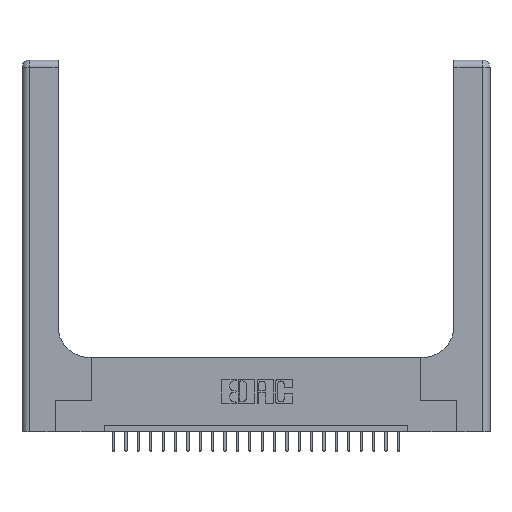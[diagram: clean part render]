
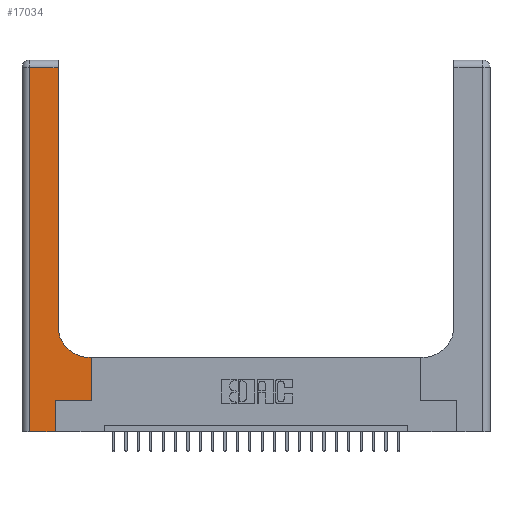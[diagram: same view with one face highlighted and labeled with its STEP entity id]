
A CAD part, top view. The second image highlights one B-rep face of the part: STEP entity #17034.
In plain terms, the highlighted planar face has unit normal (0, 0, 1).
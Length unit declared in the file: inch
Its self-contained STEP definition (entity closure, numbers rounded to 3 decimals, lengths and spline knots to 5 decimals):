
#366 = LINE ( 'NONE', #868, #18092 ) ;
#513 = DIRECTION ( 'NONE',  ( 0., 1., 0. ) ) ;
#868 = CARTESIAN_POINT ( 'NONE',  ( 0., 2.94, 0.37 ) ) ;
#1115 = EDGE_CURVE ( 'NONE', #24318, #11348, #1898, .T. ) ;
#1145 = VERTEX_POINT ( 'NONE', #16154 ) ;
#1175 = PLANE ( 'NONE',  #11330 ) ;
#1395 = LINE ( 'NONE', #10320, #18798 ) ;
#1799 = VECTOR ( 'NONE', #15553, 39.37008 ) ;
#1898 = LINE ( 'NONE', #23391, #19881 ) ;
#1941 = VERTEX_POINT ( 'NONE', #11925 ) ;
#1975 = CARTESIAN_POINT ( 'NONE',  ( 0.06, 2.94, 0.37 ) ) ;
#2392 = VERTEX_POINT ( 'NONE', #14269 ) ;
#2395 = CARTESIAN_POINT ( 'NONE',  ( 0.5415, 0.6, 0.37 ) ) ;
#2659 = ORIENTED_EDGE ( 'NONE', *, *, #9084, .T. ) ;
#3043 = LINE ( 'NONE', #3652, #1799 ) ;
#3112 = ORIENTED_EDGE ( 'NONE', *, *, #6269, .T. ) ;
#3192 = CIRCLE ( 'NONE', #4541, 0.25 ) ;
#3473 = CARTESIAN_POINT ( 'NONE',  ( 0.269, 0.25, 0.37 ) ) ;
#3652 = CARTESIAN_POINT ( 'NONE',  ( 0.269, 0., 0.37 ) ) ;
#3776 = CARTESIAN_POINT ( 'NONE',  ( 0., 0., 0.37 ) ) ;
#4541 = AXIS2_PLACEMENT_3D ( 'NONE', #4554, #4646, #24519 ) ;
#4554 = CARTESIAN_POINT ( 'NONE',  ( 0.5415, 0.85, 0.37 ) ) ;
#4646 = DIRECTION ( 'NONE',  ( 0., 0., -1. ) ) ;
#4656 = ORIENTED_EDGE ( 'NONE', *, *, #1115, .T. ) ;
#5055 = CARTESIAN_POINT ( 'NONE',  ( 0.5585, 0.25, 0.37 ) ) ;
#5147 = CARTESIAN_POINT ( 'NONE',  ( 0.2915, 0.6, 0.37 ) ) ;
#5500 = ORIENTED_EDGE ( 'NONE', *, *, #11377, .T. ) ;
#6269 = EDGE_CURVE ( 'NONE', #19962, #1941, #1395, .T. ) ;
#7213 = DIRECTION ( 'NONE',  ( 0., 1., 0. ) ) ;
#7850 = LINE ( 'NONE', #3776, #21528 ) ;
#7855 = VECTOR ( 'NONE', #7213, 39.37008 ) ;
#8507 = ORIENTED_EDGE ( 'NONE', *, *, #16821, .T. ) ;
#9084 = EDGE_CURVE ( 'NONE', #22140, #24662, #3192, .T. ) ;
#9133 = DIRECTION ( 'NONE',  ( 1., 0., 0. ) ) ;
#10320 = CARTESIAN_POINT ( 'NONE',  ( 0.5585, 0.25, 0.37 ) ) ;
#11205 = EDGE_LOOP ( 'NONE', ( #14551, #14239, #4656, #8507, #25707, #5500, #3112, #23960, #2659 ) ) ;
#11330 = AXIS2_PLACEMENT_3D ( 'NONE', #13000, #16996, #24773 ) ;
#11348 = VERTEX_POINT ( 'NONE', #12780 ) ;
#11377 = EDGE_CURVE ( 'NONE', #2392, #19962, #21696, .T. ) ;
#11525 = DIRECTION ( 'NONE',  ( 1., 0., 0. ) ) ;
#11925 = CARTESIAN_POINT ( 'NONE',  ( 0.5585, 0.6, 0.37 ) ) ;
#12433 = EDGE_CURVE ( 'NONE', #1145, #2392, #3043, .T. ) ;
#12780 = CARTESIAN_POINT ( 'NONE',  ( 0.06, 0., 0.37 ) ) ;
#12856 = DIRECTION ( 'NONE',  ( -1., 0., 0. ) ) ;
#13000 = CARTESIAN_POINT ( 'NONE',  ( 0., 3., 0.37 ) ) ;
#13415 = CARTESIAN_POINT ( 'NONE',  ( 0.2915, 2.94, 0.37 ) ) ;
#13504 = FACE_OUTER_BOUND ( 'NONE', #11205, .T. ) ;
#14239 = ORIENTED_EDGE ( 'NONE', *, *, #17835, .T. ) ;
#14269 = CARTESIAN_POINT ( 'NONE',  ( 0.269, 0.25, 0.37 ) ) ;
#14551 = ORIENTED_EDGE ( 'NONE', *, *, #22501, .T. ) ;
#14830 = DIRECTION ( 'NONE',  ( -1., 0., 0. ) ) ;
#15553 = DIRECTION ( 'NONE',  ( 0., 1., 0. ) ) ;
#16154 = CARTESIAN_POINT ( 'NONE',  ( 0.269, 0., 0.37 ) ) ;
#16480 = VECTOR ( 'NONE', #9133, 39.37008 ) ;
#16821 = EDGE_CURVE ( 'NONE', #11348, #1145, #7850, .T. ) ;
#16996 = DIRECTION ( 'NONE',  ( 0., 0., -1. ) ) ;
#17029 = EDGE_CURVE ( 'NONE', #1941, #22140, #18476, .T. ) ;
#17034 = ADVANCED_FACE ( 'NONE', ( #13504 ), #1175, .F. ) ;
#17512 = DIRECTION ( 'NONE',  ( 0., -1., 0. ) ) ;
#17806 = LINE ( 'NONE', #21030, #7855 ) ;
#17835 = EDGE_CURVE ( 'NONE', #17899, #24318, #366, .T. ) ;
#17899 = VERTEX_POINT ( 'NONE', #13415 ) ;
#18092 = VECTOR ( 'NONE', #12856, 39.37008 ) ;
#18476 = LINE ( 'NONE', #5147, #18784 ) ;
#18710 = CARTESIAN_POINT ( 'NONE',  ( 0.2915, 0.85, 0.37 ) ) ;
#18784 = VECTOR ( 'NONE', #14830, 39.37008 ) ;
#18798 = VECTOR ( 'NONE', #513, 39.37008 ) ;
#19881 = VECTOR ( 'NONE', #17512, 39.37008 ) ;
#19962 = VERTEX_POINT ( 'NONE', #5055 ) ;
#21030 = CARTESIAN_POINT ( 'NONE',  ( 0.2915, 3., 0.37 ) ) ;
#21528 = VECTOR ( 'NONE', #11525, 39.37008 ) ;
#21696 = LINE ( 'NONE', #3473, #16480 ) ;
#22140 = VERTEX_POINT ( 'NONE', #2395 ) ;
#22501 = EDGE_CURVE ( 'NONE', #24662, #17899, #17806, .T. ) ;
#23391 = CARTESIAN_POINT ( 'NONE',  ( 0.06, 3., 0.37 ) ) ;
#23960 = ORIENTED_EDGE ( 'NONE', *, *, #17029, .T. ) ;
#24318 = VERTEX_POINT ( 'NONE', #1975 ) ;
#24519 = DIRECTION ( 'NONE',  ( 1., 0., 0. ) ) ;
#24662 = VERTEX_POINT ( 'NONE', #18710 ) ;
#24773 = DIRECTION ( 'NONE',  ( -1., 0., 0. ) ) ;
#25707 = ORIENTED_EDGE ( 'NONE', *, *, #12433, .T. ) ;
